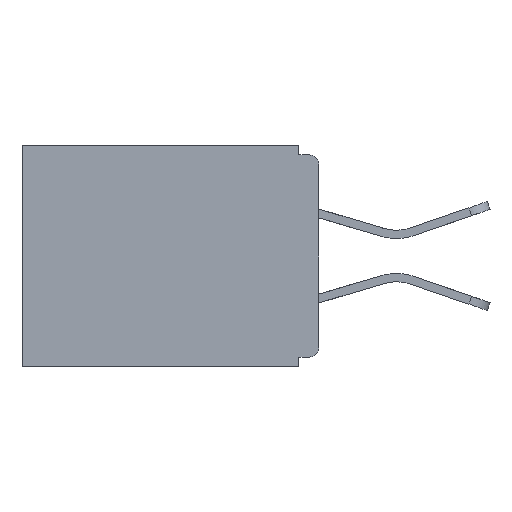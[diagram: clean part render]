
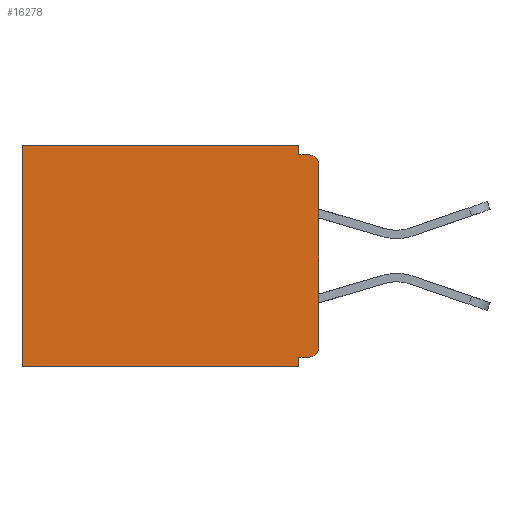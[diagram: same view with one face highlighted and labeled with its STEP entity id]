
A CAD part, left-side view. The second image highlights one B-rep face of the part: STEP entity #16278.
In plain terms, the highlighted planar face has unit normal (-1, 0, 0).
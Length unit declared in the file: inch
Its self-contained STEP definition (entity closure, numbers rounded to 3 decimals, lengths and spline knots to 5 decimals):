
#721 = VERTEX_POINT ( 'NONE', #6547 ) ;
#796 = ORIENTED_EDGE ( 'NONE', *, *, #16606, .F. ) ;
#981 = LINE ( 'NONE', #1464, #25063 ) ;
#1284 = CARTESIAN_POINT ( 'NONE',  ( 0.298, 0.46, 0. ) ) ;
#1464 = CARTESIAN_POINT ( 'NONE',  ( 0.298, 0.46, 0. ) ) ;
#1923 = CARTESIAN_POINT ( 'NONE',  ( 0.298, 0.015, -0.03 ) ) ;
#1949 = CARTESIAN_POINT ( 'NONE',  ( 0.298, 0.031, -0.328 ) ) ;
#2166 = PLANE ( 'NONE',  #10794 ) ;
#2249 = VERTEX_POINT ( 'NONE', #19348 ) ;
#2832 = LINE ( 'NONE', #7301, #7641 ) ;
#3350 = CARTESIAN_POINT ( 'NONE',  ( 0.298, 0., -0.343 ) ) ;
#3743 = ORIENTED_EDGE ( 'NONE', *, *, #25215, .T. ) ;
#3763 = EDGE_LOOP ( 'NONE', ( #24138, #8786, #24287, #16172, #3743, #796, #5681, #23395, #17936, #13811 ) ) ;
#3789 = CARTESIAN_POINT ( 'NONE',  ( 0.298, 0., -0.328 ) ) ;
#4770 = VERTEX_POINT ( 'NONE', #23524 ) ;
#5637 = VERTEX_POINT ( 'NONE', #10235 ) ;
#5681 = ORIENTED_EDGE ( 'NONE', *, *, #23044, .F. ) ;
#5853 = CARTESIAN_POINT ( 'NONE',  ( 0.298, 0., 0. ) ) ;
#6091 = LINE ( 'NONE', #5853, #14125 ) ;
#6547 = CARTESIAN_POINT ( 'NONE',  ( 0.298, 0., -0.313 ) ) ;
#7190 = DIRECTION ( 'NONE',  ( 0., 0., -1. ) ) ;
#7210 = VECTOR ( 'NONE', #23734, 39.37008 ) ;
#7266 = DIRECTION ( 'NONE',  ( 0., 0., -1. ) ) ;
#7301 = CARTESIAN_POINT ( 'NONE',  ( 0.298, 0., -0.015 ) ) ;
#7485 = CARTESIAN_POINT ( 'NONE',  ( 0.298, 0.031, -0.343 ) ) ;
#7641 = VECTOR ( 'NONE', #23728, 39.37008 ) ;
#7932 = VECTOR ( 'NONE', #7266, 39.37008 ) ;
#8286 = DIRECTION ( 'NONE',  ( 0., 1., 0. ) ) ;
#8307 = DIRECTION ( 'NONE',  ( 0., 0., -1. ) ) ;
#8411 = CIRCLE ( 'NONE', #26439, 0.015 ) ;
#8786 = ORIENTED_EDGE ( 'NONE', *, *, #10559, .F. ) ;
#8834 = EDGE_CURVE ( 'NONE', #4770, #721, #8411, .T. ) ;
#9367 = VERTEX_POINT ( 'NONE', #14895 ) ;
#9474 = CARTESIAN_POINT ( 'NONE',  ( 0.298, 0., -0.03 ) ) ;
#10235 = CARTESIAN_POINT ( 'NONE',  ( 0.298, 0.015, -0.015 ) ) ;
#10368 = VECTOR ( 'NONE', #8286, 39.37008 ) ;
#10559 = EDGE_CURVE ( 'NONE', #15224, #5637, #2832, .T. ) ;
#10638 = VERTEX_POINT ( 'NONE', #1284 ) ;
#10779 = LINE ( 'NONE', #16287, #18804 ) ;
#10794 = AXIS2_PLACEMENT_3D ( 'NONE', #12227, #16543, #14295 ) ;
#11178 = EDGE_CURVE ( 'NONE', #2249, #15224, #24276, .T. ) ;
#11942 = DIRECTION ( 'NONE',  ( 0., 0., -1. ) ) ;
#12227 = CARTESIAN_POINT ( 'NONE',  ( 0.298, 0., 0. ) ) ;
#12377 = VERTEX_POINT ( 'NONE', #9474 ) ;
#13264 = DIRECTION ( 'NONE',  ( -1., 0., 0. ) ) ;
#13811 = ORIENTED_EDGE ( 'NONE', *, *, #18433, .F. ) ;
#14125 = VECTOR ( 'NONE', #11942, 39.37008 ) ;
#14295 = DIRECTION ( 'NONE',  ( 0., 0., -1. ) ) ;
#14885 = VECTOR ( 'NONE', #23721, 39.37008 ) ;
#14895 = CARTESIAN_POINT ( 'NONE',  ( 0.298, 0.46, -0.343 ) ) ;
#15224 = VERTEX_POINT ( 'NONE', #21839 ) ;
#15261 = EDGE_CURVE ( 'NONE', #2249, #10638, #10779, .T. ) ;
#15437 = VERTEX_POINT ( 'NONE', #16816 ) ;
#15448 = CIRCLE ( 'NONE', #21818, 0.015 ) ;
#16172 = ORIENTED_EDGE ( 'NONE', *, *, #15261, .T. ) ;
#16278 = ADVANCED_FACE ( 'NONE', ( #22293 ), #2166, .F. ) ;
#16287 = CARTESIAN_POINT ( 'NONE',  ( 0.298, 0., 0. ) ) ;
#16543 = DIRECTION ( 'NONE',  ( 1., 0., 0. ) ) ;
#16606 = EDGE_CURVE ( 'NONE', #15437, #9367, #20335, .T. ) ;
#16816 = CARTESIAN_POINT ( 'NONE',  ( 0.298, 0.031, -0.343 ) ) ;
#17379 = EDGE_CURVE ( 'NONE', #4770, #22681, #24448, .T. ) ;
#17936 = ORIENTED_EDGE ( 'NONE', *, *, #8834, .T. ) ;
#17965 = EDGE_CURVE ( 'NONE', #12377, #5637, #15448, .T. ) ;
#18433 = EDGE_CURVE ( 'NONE', #12377, #721, #6091, .T. ) ;
#18804 = VECTOR ( 'NONE', #24685, 39.37008 ) ;
#19305 = CARTESIAN_POINT ( 'NONE',  ( 0.298, 0.031, -0.343 ) ) ;
#19348 = CARTESIAN_POINT ( 'NONE',  ( 0.298, 0.031, 0. ) ) ;
#20335 = LINE ( 'NONE', #3350, #14885 ) ;
#21818 = AXIS2_PLACEMENT_3D ( 'NONE', #1923, #26587, #8307 ) ;
#21839 = CARTESIAN_POINT ( 'NONE',  ( 0.298, 0.031, -0.015 ) ) ;
#22293 = FACE_OUTER_BOUND ( 'NONE', #3763, .T. ) ;
#22681 = VERTEX_POINT ( 'NONE', #1949 ) ;
#23044 = EDGE_CURVE ( 'NONE', #22681, #15437, #25818, .T. ) ;
#23395 = ORIENTED_EDGE ( 'NONE', *, *, #17379, .F. ) ;
#23524 = CARTESIAN_POINT ( 'NONE',  ( 0.298, 0.015, -0.328 ) ) ;
#23721 = DIRECTION ( 'NONE',  ( 0., 1., 0. ) ) ;
#23728 = DIRECTION ( 'NONE',  ( 0., -1., 0. ) ) ;
#23734 = DIRECTION ( 'NONE',  ( 0., 0., -1. ) ) ;
#23752 = DIRECTION ( 'NONE',  ( 0., 0., -1. ) ) ;
#24138 = ORIENTED_EDGE ( 'NONE', *, *, #17965, .T. ) ;
#24276 = LINE ( 'NONE', #19305, #7932 ) ;
#24287 = ORIENTED_EDGE ( 'NONE', *, *, #11178, .F. ) ;
#24448 = LINE ( 'NONE', #3789, #10368 ) ;
#24685 = DIRECTION ( 'NONE',  ( 0., 1., 0. ) ) ;
#25063 = VECTOR ( 'NONE', #7190, 39.37008 ) ;
#25215 = EDGE_CURVE ( 'NONE', #10638, #9367, #981, .T. ) ;
#25533 = CARTESIAN_POINT ( 'NONE',  ( 0.298, 0.015, -0.313 ) ) ;
#25818 = LINE ( 'NONE', #7485, #7210 ) ;
#26439 = AXIS2_PLACEMENT_3D ( 'NONE', #25533, #13264, #23752 ) ;
#26587 = DIRECTION ( 'NONE',  ( -1., 0., 0. ) ) ;
